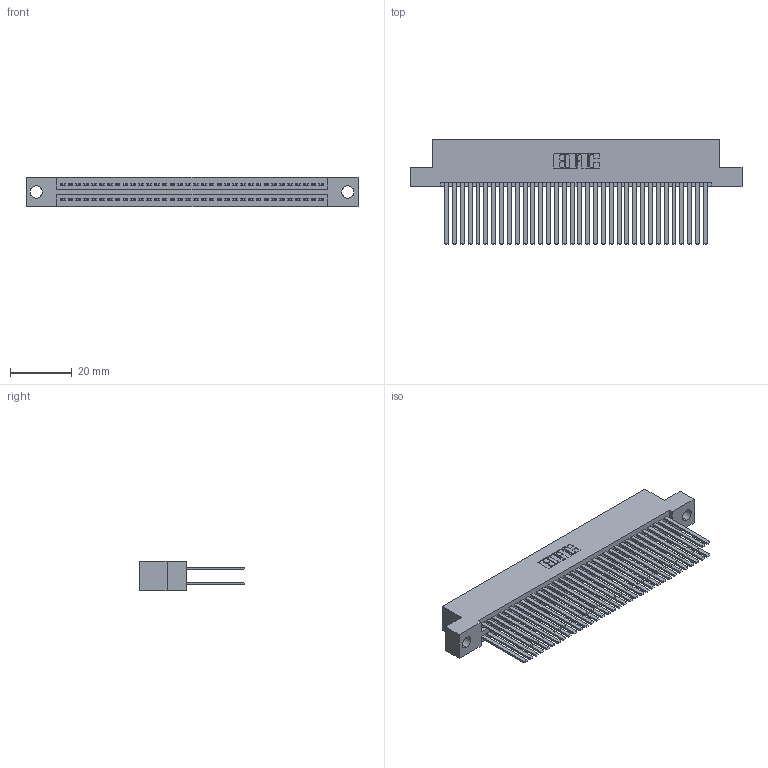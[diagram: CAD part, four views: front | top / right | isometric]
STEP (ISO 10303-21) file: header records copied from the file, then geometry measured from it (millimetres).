
FILE_DESCRIPTION (( 'STEP AP203' ), '1' );
FILE_NAME ('345-068-544-204.STEP', '2021-05-20T07:49:39', ( '' ), ( '' ), 'SwSTEP 2.0', 'SolidWorks 2020', '' );
FILE_SCHEMA (( 'CONFIG_CONTROL_DESIGN' ));
Length unit declared in the file: inch
Products named in the file (3): 345-068-544-204; 345 Part_Flush Mounting Lugs - 0.156 Dia-TI; 345-292-001_345-293-144
Assembly tree (69 placements, depth 2):
  345-068-544-204
    345 Part_Flush Mounting Lugs - 0.156 Dia-TI
    345-292-001_345-293-144  x68
Bounding box: 107.57 x 33.96 x 9.4 mm (x, y, z)
Volume: 11222.4 mm3; surface area: 19079.1 mm2
Topology: 69 solids, 69 shells, 3132 faces, 9285 edges, 6098 vertices
Faces by surface type: plane 2066, cylinder 1066
Entity records: 27989 total; most frequent: CARTESIAN_POINT 4702, ORIENTED_EDGE 4634, DIRECTION 4153, EDGE_CURVE 2317, LINE 2053, VECTOR 2053, VERTEX_POINT 1542, AXIS2_PLACEMENT_3D 1050
